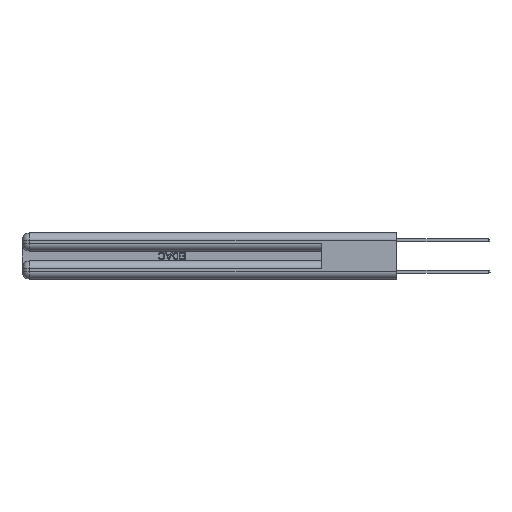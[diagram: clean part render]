
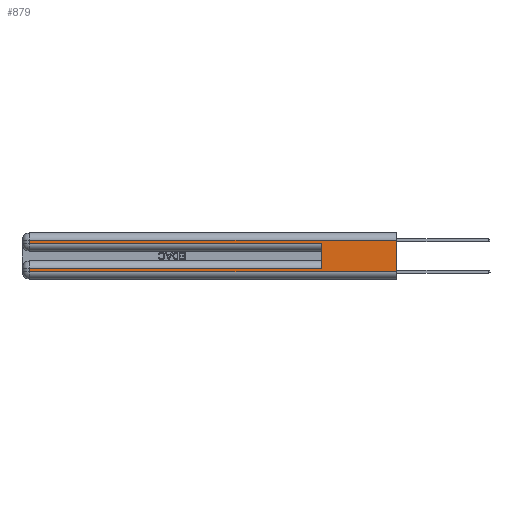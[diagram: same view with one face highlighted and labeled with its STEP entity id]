
A CAD part, left-side view. The second image highlights one B-rep face of the part: STEP entity #879.
In plain terms, the highlighted planar face has unit normal (-1, 0, 0).
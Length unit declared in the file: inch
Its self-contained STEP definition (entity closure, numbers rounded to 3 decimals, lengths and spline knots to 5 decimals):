
#69 = ORIENTED_EDGE ( 'NONE', *, *, #29910, .T. ) ;
#265 = ORIENTED_EDGE ( 'NONE', *, *, #18368, .T. ) ;
#348 = EDGE_CURVE ( 'NONE', #23963, #30588, #13665, .T. ) ;
#402 = CARTESIAN_POINT ( 'NONE',  ( 0., 0., 0.37 ) ) ;
#804 = CARTESIAN_POINT ( 'NONE',  ( 0., 2.94, 0.085 ) ) ;
#879 = ADVANCED_FACE ( 'NONE', ( #8867 ), #12535, .F. ) ;
#928 = VECTOR ( 'NONE', #24604, 39.37008 ) ;
#1714 = DIRECTION ( 'NONE',  ( 0., 0., 1. ) ) ;
#1882 = ORIENTED_EDGE ( 'NONE', *, *, #9762, .T. ) ;
#1927 = EDGE_CURVE ( 'NONE', #19783, #32177, #32878, .T. ) ;
#2107 = LINE ( 'NONE', #26419, #928 ) ;
#3899 = CARTESIAN_POINT ( 'NONE',  ( 0., 2.94, 0.31 ) ) ;
#3983 = ORIENTED_EDGE ( 'NONE', *, *, #1927, .F. ) ;
#6230 = VERTEX_POINT ( 'NONE', #3899 ) ;
#6450 = CARTESIAN_POINT ( 'NONE',  ( 0., 0.6, 0.145 ) ) ;
#7472 = CARTESIAN_POINT ( 'NONE',  ( 0., 0., 0.31 ) ) ;
#8009 = CARTESIAN_POINT ( 'NONE',  ( 0., 0.6, 0.285 ) ) ;
#8134 = DIRECTION ( 'NONE',  ( 0., -1., 0. ) ) ;
#8254 = CARTESIAN_POINT ( 'NONE',  ( 0., 0., 0.06 ) ) ;
#8503 = CARTESIAN_POINT ( 'NONE',  ( 0., 2.94, 0.37 ) ) ;
#8867 = FACE_OUTER_BOUND ( 'NONE', #31849, .T. ) ;
#9143 = VERTEX_POINT ( 'NONE', #17105 ) ;
#9283 = ORIENTED_EDGE ( 'NONE', *, *, #16253, .T. ) ;
#9762 = EDGE_CURVE ( 'NONE', #23963, #27818, #26430, .T. ) ;
#10186 = ORIENTED_EDGE ( 'NONE', *, *, #19002, .T. ) ;
#11143 = CARTESIAN_POINT ( 'NONE',  ( 0., 2.94, 0.37 ) ) ;
#12535 = PLANE ( 'NONE',  #27840 ) ;
#13028 = LINE ( 'NONE', #11143, #23864 ) ;
#13329 = DIRECTION ( 'NONE',  ( 0., 0., -1. ) ) ;
#13661 = LINE ( 'NONE', #8503, #20900 ) ;
#13665 = LINE ( 'NONE', #6450, #23660 ) ;
#13668 = CARTESIAN_POINT ( 'NONE',  ( 0., 0., 0.285 ) ) ;
#13680 = DIRECTION ( 'NONE',  ( 0., 1., 0. ) ) ;
#14920 = VECTOR ( 'NONE', #8134, 39.37008 ) ;
#14936 = CARTESIAN_POINT ( 'NONE',  ( 0., 2.94, 0.06 ) ) ;
#15203 = CARTESIAN_POINT ( 'NONE',  ( 0., 0., 0.37 ) ) ;
#15419 = DIRECTION ( 'NONE',  ( 0., 0., -1. ) ) ;
#15837 = DIRECTION ( 'NONE',  ( 0., 0., -1. ) ) ;
#16253 = EDGE_CURVE ( 'NONE', #6230, #9143, #13028, .T. ) ;
#16373 = DIRECTION ( 'NONE',  ( 0., -1., 0. ) ) ;
#17105 = CARTESIAN_POINT ( 'NONE',  ( 0., 2.94, 0.285 ) ) ;
#18368 = EDGE_CURVE ( 'NONE', #26493, #32177, #22555, .T. ) ;
#18486 = DIRECTION ( 'NONE',  ( 0., 0., -1. ) ) ;
#18837 = EDGE_CURVE ( 'NONE', #9143, #30588, #22114, .T. ) ;
#19002 = EDGE_CURVE ( 'NONE', #19783, #6230, #2107, .T. ) ;
#19783 = VERTEX_POINT ( 'NONE', #7472 ) ;
#19830 = CARTESIAN_POINT ( 'NONE',  ( 0., 0., 0.06 ) ) ;
#20900 = VECTOR ( 'NONE', #15837, 39.37008 ) ;
#21221 = VECTOR ( 'NONE', #13329, 39.37008 ) ;
#21454 = CARTESIAN_POINT ( 'NONE',  ( 0., 0.6, 0.085 ) ) ;
#22114 = LINE ( 'NONE', #13668, #30141 ) ;
#22555 = LINE ( 'NONE', #8254, #14920 ) ;
#23660 = VECTOR ( 'NONE', #1714, 39.37008 ) ;
#23864 = VECTOR ( 'NONE', #18486, 39.37008 ) ;
#23963 = VERTEX_POINT ( 'NONE', #21454 ) ;
#24604 = DIRECTION ( 'NONE',  ( 0., 1., 0. ) ) ;
#26419 = CARTESIAN_POINT ( 'NONE',  ( 0., 0., 0.31 ) ) ;
#26430 = LINE ( 'NONE', #26470, #31255 ) ;
#26470 = CARTESIAN_POINT ( 'NONE',  ( 0., 0., 0.085 ) ) ;
#26493 = VERTEX_POINT ( 'NONE', #14936 ) ;
#27818 = VERTEX_POINT ( 'NONE', #804 ) ;
#27840 = AXIS2_PLACEMENT_3D ( 'NONE', #15203, #27880, #15419 ) ;
#27880 = DIRECTION ( 'NONE',  ( 1., 0., 0. ) ) ;
#27882 = ORIENTED_EDGE ( 'NONE', *, *, #18837, .T. ) ;
#28721 = ORIENTED_EDGE ( 'NONE', *, *, #348, .F. ) ;
#29910 = EDGE_CURVE ( 'NONE', #27818, #26493, #13661, .T. ) ;
#30141 = VECTOR ( 'NONE', #16373, 39.37008 ) ;
#30588 = VERTEX_POINT ( 'NONE', #8009 ) ;
#31255 = VECTOR ( 'NONE', #13680, 39.37008 ) ;
#31849 = EDGE_LOOP ( 'NONE', ( #3983, #10186, #9283, #27882, #28721, #1882, #69, #265 ) ) ;
#32177 = VERTEX_POINT ( 'NONE', #19830 ) ;
#32878 = LINE ( 'NONE', #402, #21221 ) ;
